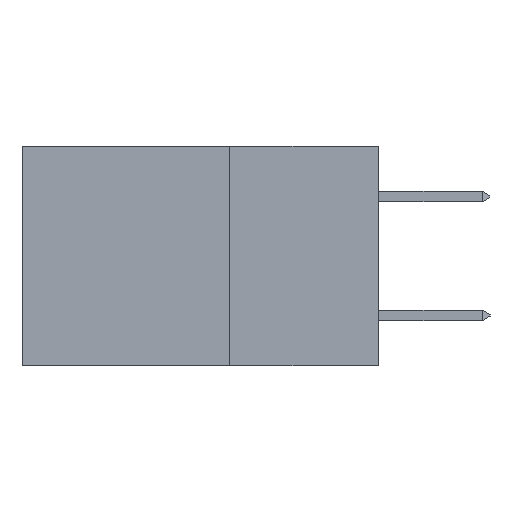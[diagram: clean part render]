
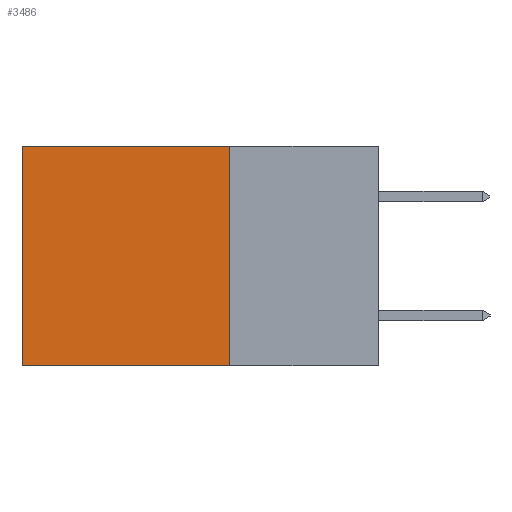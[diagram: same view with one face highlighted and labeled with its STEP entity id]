
A CAD part, left-side view. The second image highlights one B-rep face of the part: STEP entity #3486.
In plain terms, the highlighted planar face has unit normal (-1, 0, 0).
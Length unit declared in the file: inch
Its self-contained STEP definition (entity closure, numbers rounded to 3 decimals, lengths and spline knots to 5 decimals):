
#610 = EDGE_LOOP ( 'NONE', ( #11188, #7889, #11860, #9559 ) ) ;
#789 = CARTESIAN_POINT ( 'NONE',  ( 0.2615, 0.25, -0.37 ) ) ;
#1415 = DIRECTION ( 'NONE',  ( 0., 0., -1. ) ) ;
#2205 = VECTOR ( 'NONE', #9207, 39.37008 ) ;
#2359 = VERTEX_POINT ( 'NONE', #12450 ) ;
#2854 = VECTOR ( 'NONE', #11477, 39.37008 ) ;
#2890 = VECTOR ( 'NONE', #1415, 39.37008 ) ;
#3140 = FACE_OUTER_BOUND ( 'NONE', #610, .T. ) ;
#3486 = ADVANCED_FACE ( 'NONE', ( #3140 ), #8615, .F. ) ;
#3745 = CARTESIAN_POINT ( 'NONE',  ( 0.2615, 0.6, -0.37 ) ) ;
#4096 = CARTESIAN_POINT ( 'NONE',  ( 0.2615, 0.6, -0.37 ) ) ;
#4305 = CARTESIAN_POINT ( 'NONE',  ( 0.2615, 0.25, -0.37 ) ) ;
#4711 = CARTESIAN_POINT ( 'NONE',  ( 0.2615, 0.25, 0. ) ) ;
#5012 = CARTESIAN_POINT ( 'NONE',  ( 0.2615, 0.25, -0.37 ) ) ;
#5223 = EDGE_CURVE ( 'NONE', #2359, #12435, #5848, .T. ) ;
#5274 = EDGE_CURVE ( 'NONE', #13016, #5484, #11238, .T. ) ;
#5484 = VERTEX_POINT ( 'NONE', #4096 ) ;
#5848 = LINE ( 'NONE', #12198, #2890 ) ;
#6013 = EDGE_CURVE ( 'NONE', #12435, #5484, #6158, .T. ) ;
#6158 = LINE ( 'NONE', #5012, #2854 ) ;
#6446 = DIRECTION ( 'NONE',  ( 1., 0., 0. ) ) ;
#7889 = ORIENTED_EDGE ( 'NONE', *, *, #6013, .F. ) ;
#7923 = VECTOR ( 'NONE', #10126, 39.37008 ) ;
#8615 = PLANE ( 'NONE',  #9542 ) ;
#9207 = DIRECTION ( 'NONE',  ( 0., 0., -1. ) ) ;
#9542 = AXIS2_PLACEMENT_3D ( 'NONE', #789, #6446, #13764 ) ;
#9559 = ORIENTED_EDGE ( 'NONE', *, *, #11219, .T. ) ;
#10126 = DIRECTION ( 'NONE',  ( 0., 1., 0. ) ) ;
#11073 = LINE ( 'NONE', #4711, #7923 ) ;
#11188 = ORIENTED_EDGE ( 'NONE', *, *, #5274, .T. ) ;
#11219 = EDGE_CURVE ( 'NONE', #2359, #13016, #11073, .T. ) ;
#11238 = LINE ( 'NONE', #3745, #2205 ) ;
#11477 = DIRECTION ( 'NONE',  ( 0., 1., 0. ) ) ;
#11860 = ORIENTED_EDGE ( 'NONE', *, *, #5223, .F. ) ;
#12198 = CARTESIAN_POINT ( 'NONE',  ( 0.2615, 0.25, -0.37 ) ) ;
#12435 = VERTEX_POINT ( 'NONE', #4305 ) ;
#12450 = CARTESIAN_POINT ( 'NONE',  ( 0.2615, 0.25, 0. ) ) ;
#13016 = VERTEX_POINT ( 'NONE', #13631 ) ;
#13631 = CARTESIAN_POINT ( 'NONE',  ( 0.2615, 0.6, 0. ) ) ;
#13764 = DIRECTION ( 'NONE',  ( 0., 0., -1. ) ) ;
